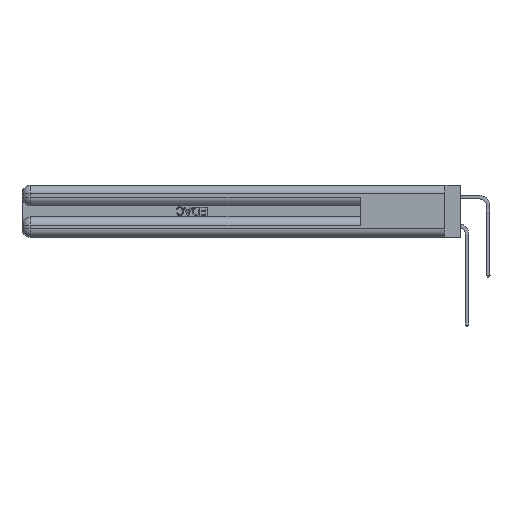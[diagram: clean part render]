
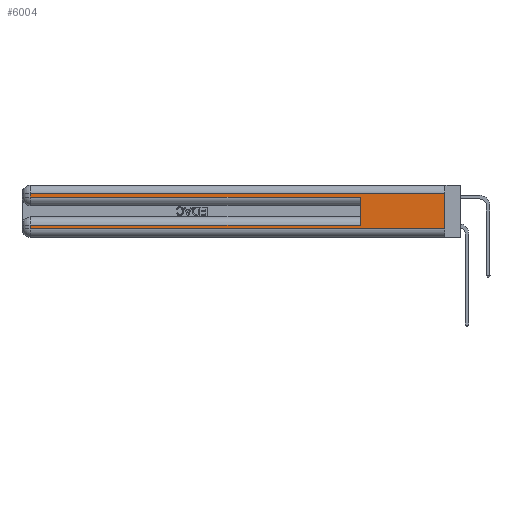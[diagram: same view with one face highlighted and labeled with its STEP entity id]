
A CAD part, left-side view. The second image highlights one B-rep face of the part: STEP entity #6004.
In plain terms, the highlighted planar face has unit normal (-1, 0, 0).
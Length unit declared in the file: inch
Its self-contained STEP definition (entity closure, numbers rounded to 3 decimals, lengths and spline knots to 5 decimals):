
#372 = ORIENTED_EDGE ( 'NONE', *, *, #29537, .F. ) ;
#1409 = CARTESIAN_POINT ( 'NONE',  ( 0., 0., 0.31 ) ) ;
#1693 = CARTESIAN_POINT ( 'NONE',  ( 0., 0.6, 0.285 ) ) ;
#1827 = DIRECTION ( 'NONE',  ( 0., 0., -1. ) ) ;
#1867 = CARTESIAN_POINT ( 'NONE',  ( 0., 0., 0.06 ) ) ;
#2320 = CARTESIAN_POINT ( 'NONE',  ( 0., 0., 0.06 ) ) ;
#3599 = EDGE_LOOP ( 'NONE', ( #372, #35333, #28746, #29760, #23101, #6578, #7624, #17447 ) ) ;
#4642 = CARTESIAN_POINT ( 'NONE',  ( 0., 0., 0.285 ) ) ;
#4907 = VECTOR ( 'NONE', #35626, 39.37008 ) ;
#6004 = ADVANCED_FACE ( 'NONE', ( #23755 ), #11620, .F. ) ;
#6578 = ORIENTED_EDGE ( 'NONE', *, *, #14263, .T. ) ;
#6616 = VECTOR ( 'NONE', #39319, 39.37008 ) ;
#7213 = EDGE_CURVE ( 'NONE', #7387, #17889, #39479, .T. ) ;
#7387 = VERTEX_POINT ( 'NONE', #1409 ) ;
#7624 = ORIENTED_EDGE ( 'NONE', *, *, #21495, .T. ) ;
#7943 = DIRECTION ( 'NONE',  ( 0., -1., 0. ) ) ;
#8826 = VECTOR ( 'NONE', #18623, 39.37008 ) ;
#9535 = CARTESIAN_POINT ( 'NONE',  ( 0., 0., 0.37 ) ) ;
#9626 = VECTOR ( 'NONE', #38136, 39.37008 ) ;
#9866 = LINE ( 'NONE', #41519, #8826 ) ;
#11620 = PLANE ( 'NONE',  #16173 ) ;
#12267 = DIRECTION ( 'NONE',  ( 0., -1., 0. ) ) ;
#14263 = EDGE_CURVE ( 'NONE', #26831, #20124, #9866, .T. ) ;
#15810 = VERTEX_POINT ( 'NONE', #26821 ) ;
#16173 = AXIS2_PLACEMENT_3D ( 'NONE', #41156, #21561, #1827 ) ;
#17315 = VERTEX_POINT ( 'NONE', #1693 ) ;
#17447 = ORIENTED_EDGE ( 'NONE', *, *, #20073, .T. ) ;
#17713 = VECTOR ( 'NONE', #7943, 39.37008 ) ;
#17889 = VERTEX_POINT ( 'NONE', #30560 ) ;
#18401 = LINE ( 'NONE', #25154, #9626 ) ;
#18584 = CARTESIAN_POINT ( 'NONE',  ( 0., 2.94, 0.06 ) ) ;
#18623 = DIRECTION ( 'NONE',  ( 0., 1., 0. ) ) ;
#19753 = VECTOR ( 'NONE', #26046, 39.37008 ) ;
#20073 = EDGE_CURVE ( 'NONE', #25786, #24957, #31741, .T. ) ;
#20124 = VERTEX_POINT ( 'NONE', #38620 ) ;
#21495 = EDGE_CURVE ( 'NONE', #20124, #25786, #39828, .T. ) ;
#21561 = DIRECTION ( 'NONE',  ( 1., 0., 0. ) ) ;
#22655 = CARTESIAN_POINT ( 'NONE',  ( 0., 2.94, 0.37 ) ) ;
#23101 = ORIENTED_EDGE ( 'NONE', *, *, #35618, .F. ) ;
#23755 = FACE_OUTER_BOUND ( 'NONE', #3599, .T. ) ;
#24142 = EDGE_CURVE ( 'NONE', #15810, #17315, #27481, .T. ) ;
#24506 = VECTOR ( 'NONE', #32514, 39.37008 ) ;
#24957 = VERTEX_POINT ( 'NONE', #1867 ) ;
#25154 = CARTESIAN_POINT ( 'NONE',  ( 0., 2.94, 0.37 ) ) ;
#25786 = VERTEX_POINT ( 'NONE', #18584 ) ;
#26046 = DIRECTION ( 'NONE',  ( 0., 0., 1. ) ) ;
#26341 = CARTESIAN_POINT ( 'NONE',  ( 0., 0., 0.31 ) ) ;
#26821 = CARTESIAN_POINT ( 'NONE',  ( 0., 2.94, 0.285 ) ) ;
#26831 = VERTEX_POINT ( 'NONE', #29971 ) ;
#27481 = LINE ( 'NONE', #4642, #17713 ) ;
#28460 = LINE ( 'NONE', #42320, #19753 ) ;
#28746 = ORIENTED_EDGE ( 'NONE', *, *, #28798, .T. ) ;
#28798 = EDGE_CURVE ( 'NONE', #17889, #15810, #18401, .T. ) ;
#29537 = EDGE_CURVE ( 'NONE', #7387, #24957, #33175, .T. ) ;
#29760 = ORIENTED_EDGE ( 'NONE', *, *, #24142, .T. ) ;
#29971 = CARTESIAN_POINT ( 'NONE',  ( 0., 0.6, 0.085 ) ) ;
#30560 = CARTESIAN_POINT ( 'NONE',  ( 0., 2.94, 0.31 ) ) ;
#30717 = VECTOR ( 'NONE', #12267, 39.37008 ) ;
#31741 = LINE ( 'NONE', #2320, #30717 ) ;
#32514 = DIRECTION ( 'NONE',  ( 0., 0., -1. ) ) ;
#33175 = LINE ( 'NONE', #9535, #24506 ) ;
#35333 = ORIENTED_EDGE ( 'NONE', *, *, #7213, .T. ) ;
#35618 = EDGE_CURVE ( 'NONE', #26831, #17315, #28460, .T. ) ;
#35626 = DIRECTION ( 'NONE',  ( 0., 0., -1. ) ) ;
#38136 = DIRECTION ( 'NONE',  ( 0., 0., -1. ) ) ;
#38620 = CARTESIAN_POINT ( 'NONE',  ( 0., 2.94, 0.085 ) ) ;
#39319 = DIRECTION ( 'NONE',  ( 0., 1., 0. ) ) ;
#39479 = LINE ( 'NONE', #26341, #6616 ) ;
#39828 = LINE ( 'NONE', #22655, #4907 ) ;
#41156 = CARTESIAN_POINT ( 'NONE',  ( 0., 0., 0.37 ) ) ;
#41519 = CARTESIAN_POINT ( 'NONE',  ( 0., 0., 0.085 ) ) ;
#42320 = CARTESIAN_POINT ( 'NONE',  ( 0., 0.6, 0.145 ) ) ;
